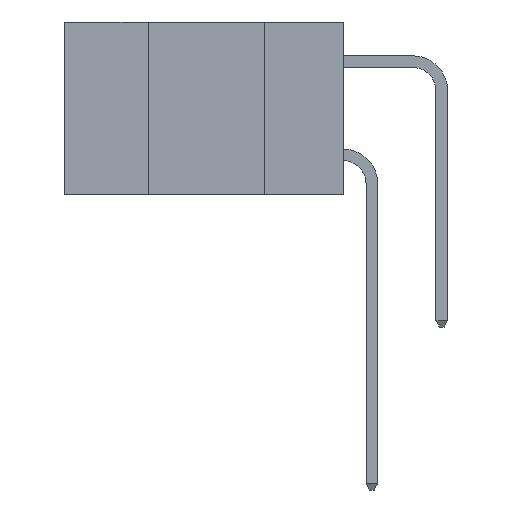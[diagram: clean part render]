
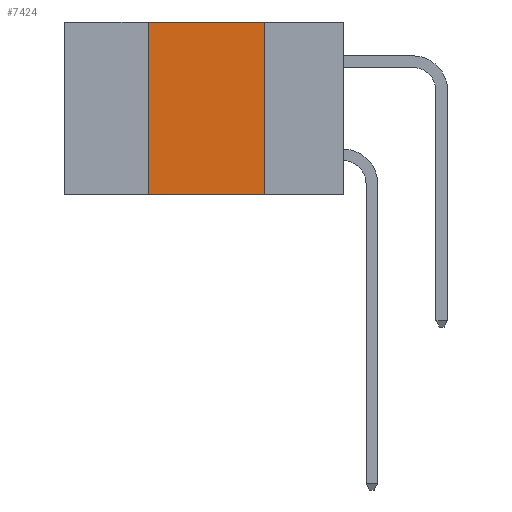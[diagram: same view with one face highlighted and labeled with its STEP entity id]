
A CAD part, left-side view. The second image highlights one B-rep face of the part: STEP entity #7424.
In plain terms, the highlighted planar face has unit normal (-1, 0, 0).
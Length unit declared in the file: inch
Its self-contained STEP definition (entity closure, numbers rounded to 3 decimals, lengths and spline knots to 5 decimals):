
#198 = CARTESIAN_POINT ( 'NONE',  ( 0., 0.6, 0. ) ) ;
#323 = ORIENTED_EDGE ( 'NONE', *, *, #3984, .F. ) ;
#1026 = CARTESIAN_POINT ( 'NONE',  ( 0., 0.17, -0.37 ) ) ;
#1099 = DIRECTION ( 'NONE',  ( 0., 0., -1. ) ) ;
#1374 = ORIENTED_EDGE ( 'NONE', *, *, #2214, .T. ) ;
#1919 = CARTESIAN_POINT ( 'NONE',  ( 0., 0.17, -0.37 ) ) ;
#2214 = EDGE_CURVE ( 'NONE', #7848, #4473, #7539, .T. ) ;
#2540 = LINE ( 'NONE', #1026, #9062 ) ;
#2805 = EDGE_CURVE ( 'NONE', #7848, #5079, #10409, .T. ) ;
#2829 = VERTEX_POINT ( 'NONE', #6312 ) ;
#3753 = DIRECTION ( 'NONE',  ( 0., 0., -1. ) ) ;
#3754 = ORIENTED_EDGE ( 'NONE', *, *, #4535, .F. ) ;
#3774 = ORIENTED_EDGE ( 'NONE', *, *, #2805, .F. ) ;
#3781 = DIRECTION ( 'NONE',  ( 0., 0., 1. ) ) ;
#3984 = EDGE_CURVE ( 'NONE', #5079, #2829, #5108, .T. ) ;
#4473 = VERTEX_POINT ( 'NONE', #1919 ) ;
#4535 = EDGE_CURVE ( 'NONE', #2829, #4473, #2540, .T. ) ;
#4580 = EDGE_LOOP ( 'NONE', ( #3754, #323, #3774, #1374 ) ) ;
#5079 = VERTEX_POINT ( 'NONE', #5221 ) ;
#5108 = LINE ( 'NONE', #198, #7525 ) ;
#5221 = CARTESIAN_POINT ( 'NONE',  ( 0., 0.42, 0. ) ) ;
#5457 = CARTESIAN_POINT ( 'NONE',  ( 0., 0.6, 0. ) ) ;
#5903 = CARTESIAN_POINT ( 'NONE',  ( 0., 0.42, -0.37 ) ) ;
#6303 = DIRECTION ( 'NONE',  ( 1., 0., 0. ) ) ;
#6312 = CARTESIAN_POINT ( 'NONE',  ( 0., 0.17, 0. ) ) ;
#6554 = CARTESIAN_POINT ( 'NONE',  ( 0., 0.6, -0.37 ) ) ;
#7300 = VECTOR ( 'NONE', #7337, 39.37008 ) ;
#7337 = DIRECTION ( 'NONE',  ( 0., -1., 0. ) ) ;
#7369 = FACE_OUTER_BOUND ( 'NONE', #4580, .T. ) ;
#7424 = ADVANCED_FACE ( 'NONE', ( #7369 ), #10134, .F. ) ;
#7525 = VECTOR ( 'NONE', #8813, 39.37008 ) ;
#7539 = LINE ( 'NONE', #6554, #7300 ) ;
#7848 = VERTEX_POINT ( 'NONE', #5903 ) ;
#7865 = CARTESIAN_POINT ( 'NONE',  ( 0., 0.42, -0.37 ) ) ;
#8139 = VECTOR ( 'NONE', #3781, 39.37008 ) ;
#8813 = DIRECTION ( 'NONE',  ( 0., -1., 0. ) ) ;
#8950 = AXIS2_PLACEMENT_3D ( 'NONE', #5457, #6303, #1099 ) ;
#9062 = VECTOR ( 'NONE', #3753, 39.37008 ) ;
#10134 = PLANE ( 'NONE',  #8950 ) ;
#10409 = LINE ( 'NONE', #7865, #8139 ) ;
